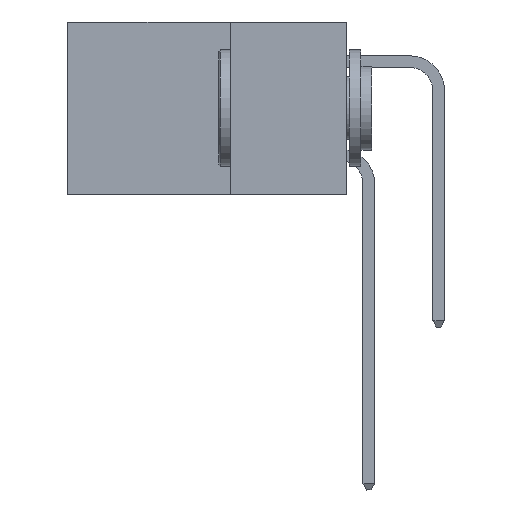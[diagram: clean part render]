
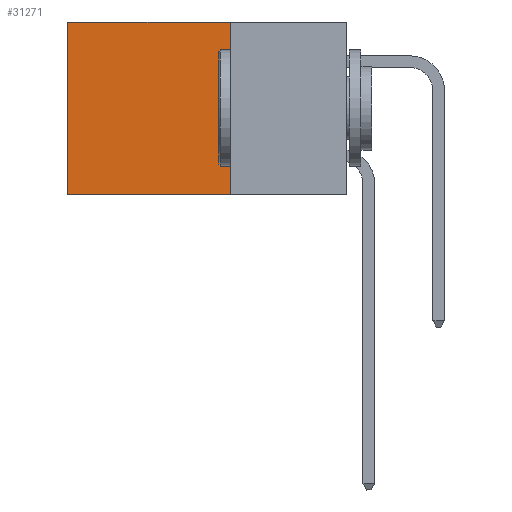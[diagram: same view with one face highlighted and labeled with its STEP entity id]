
A CAD part, left-side view. The second image highlights one B-rep face of the part: STEP entity #31271.
In plain terms, the highlighted planar face has unit normal (-1, 0, 0).
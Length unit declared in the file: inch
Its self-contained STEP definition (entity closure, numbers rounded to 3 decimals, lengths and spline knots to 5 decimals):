
#142 = AXIS2_PLACEMENT_3D ( 'NONE', #6292, #17898, #24360 ) ;
#716 = LINE ( 'NONE', #18233, #17798 ) ;
#3386 = ORIENTED_EDGE ( 'NONE', *, *, #25047, .F. ) ;
#4221 = ORIENTED_EDGE ( 'NONE', *, *, #29158, .T. ) ;
#5896 = EDGE_CURVE ( 'NONE', #21961, #19582, #716, .T. ) ;
#6292 = CARTESIAN_POINT ( 'NONE',  ( 0.2875, 0.25, 0. ) ) ;
#6764 = CARTESIAN_POINT ( 'NONE',  ( 0.2875, 0.6, 0. ) ) ;
#7693 = VECTOR ( 'NONE', #32649, 39.37008 ) ;
#8013 = DIRECTION ( 'NONE',  ( 0., 0., -1. ) ) ;
#8581 = CARTESIAN_POINT ( 'NONE',  ( 0.2875, 0.25, 0. ) ) ;
#10282 = EDGE_LOOP ( 'NONE', ( #4221, #3386, #23069, #13123 ) ) ;
#10820 = VERTEX_POINT ( 'NONE', #26257 ) ;
#12244 = LINE ( 'NONE', #6764, #21276 ) ;
#13123 = ORIENTED_EDGE ( 'NONE', *, *, #27049, .T. ) ;
#15684 = LINE ( 'NONE', #8581, #7693 ) ;
#16770 = FACE_OUTER_BOUND ( 'NONE', #10282, .T. ) ;
#17798 = VECTOR ( 'NONE', #36365, 39.37008 ) ;
#17898 = DIRECTION ( 'NONE',  ( 1., 0., 0. ) ) ;
#18233 = CARTESIAN_POINT ( 'NONE',  ( 0.2875, 0.25, 0. ) ) ;
#18517 = LINE ( 'NONE', #28533, #29862 ) ;
#19582 = VERTEX_POINT ( 'NONE', #24280 ) ;
#21276 = VECTOR ( 'NONE', #8013, 39.37008 ) ;
#21351 = PLANE ( 'NONE',  #142 ) ;
#21961 = VERTEX_POINT ( 'NONE', #31635 ) ;
#23069 = ORIENTED_EDGE ( 'NONE', *, *, #5896, .F. ) ;
#24280 = CARTESIAN_POINT ( 'NONE',  ( 0.2875, 0.25, -0.37 ) ) ;
#24360 = DIRECTION ( 'NONE',  ( 0., 0., -1. ) ) ;
#25047 = EDGE_CURVE ( 'NONE', #19582, #25703, #18517, .T. ) ;
#25322 = CARTESIAN_POINT ( 'NONE',  ( 0.2875, 0.6, -0.37 ) ) ;
#25703 = VERTEX_POINT ( 'NONE', #25322 ) ;
#26257 = CARTESIAN_POINT ( 'NONE',  ( 0.2875, 0.6, 0. ) ) ;
#27049 = EDGE_CURVE ( 'NONE', #21961, #10820, #15684, .T. ) ;
#28533 = CARTESIAN_POINT ( 'NONE',  ( 0.2875, 0.25, -0.37 ) ) ;
#29158 = EDGE_CURVE ( 'NONE', #10820, #25703, #12244, .T. ) ;
#29862 = VECTOR ( 'NONE', #31858, 39.37008 ) ;
#31271 = ADVANCED_FACE ( 'NONE', ( #16770 ), #21351, .F. ) ;
#31635 = CARTESIAN_POINT ( 'NONE',  ( 0.2875, 0.25, 0. ) ) ;
#31858 = DIRECTION ( 'NONE',  ( 0., 1., 0. ) ) ;
#32649 = DIRECTION ( 'NONE',  ( 0., 1., 0. ) ) ;
#36365 = DIRECTION ( 'NONE',  ( 0., 0., -1. ) ) ;
